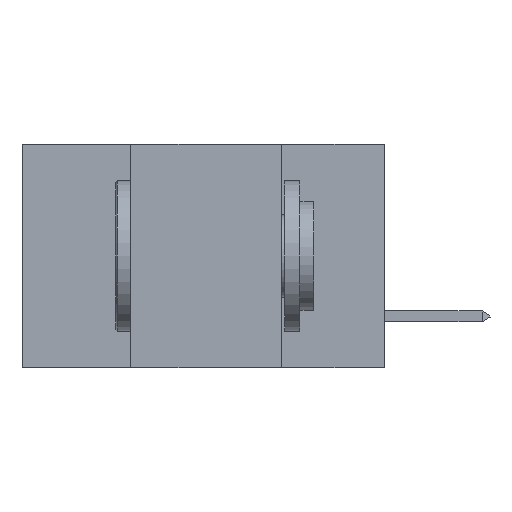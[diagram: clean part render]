
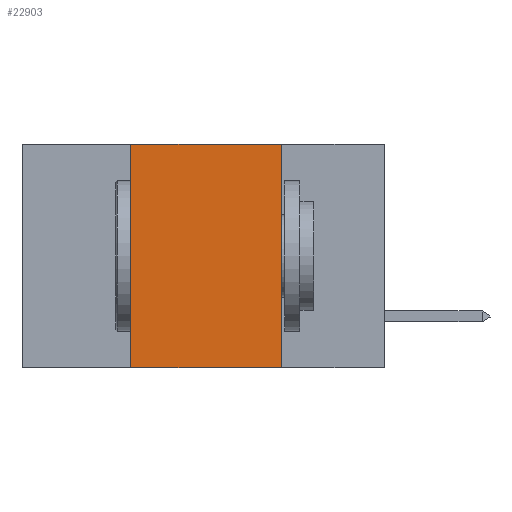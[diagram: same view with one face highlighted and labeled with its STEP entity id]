
A CAD part, left-side view. The second image highlights one B-rep face of the part: STEP entity #22903.
In plain terms, the highlighted planar face has unit normal (-1, 0, 0).
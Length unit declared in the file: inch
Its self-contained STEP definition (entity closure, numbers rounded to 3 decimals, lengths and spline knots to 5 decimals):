
#1036 = DIRECTION ( 'NONE',  ( 0., 0., -1. ) ) ;
#1181 = ORIENTED_EDGE ( 'NONE', *, *, #3146, .T. ) ;
#2586 = CARTESIAN_POINT ( 'NONE',  ( 0., 0.6, 0. ) ) ;
#2651 = CARTESIAN_POINT ( 'NONE',  ( 0., 0.17, -0.37 ) ) ;
#3146 = EDGE_CURVE ( 'NONE', #17203, #20157, #23540, .T. ) ;
#3471 = CARTESIAN_POINT ( 'NONE',  ( 0., 0.42, 0. ) ) ;
#3486 = VERTEX_POINT ( 'NONE', #8596 ) ;
#3766 = ORIENTED_EDGE ( 'NONE', *, *, #17539, .F. ) ;
#3895 = EDGE_LOOP ( 'NONE', ( #9878, #3766, #4233, #1181 ) ) ;
#4100 = CARTESIAN_POINT ( 'NONE',  ( 0., 0.42, -0.37 ) ) ;
#4233 = ORIENTED_EDGE ( 'NONE', *, *, #4370, .F. ) ;
#4370 = EDGE_CURVE ( 'NONE', #17203, #14388, #13505, .T. ) ;
#5021 = DIRECTION ( 'NONE',  ( 0., 0., -1. ) ) ;
#5562 = EDGE_CURVE ( 'NONE', #3486, #20157, #23439, .T. ) ;
#8101 = DIRECTION ( 'NONE',  ( 0., -1., 0. ) ) ;
#8596 = CARTESIAN_POINT ( 'NONE',  ( 0., 0.17, 0. ) ) ;
#8772 = VECTOR ( 'NONE', #1036, 39.37008 ) ;
#8903 = DIRECTION ( 'NONE',  ( 1., 0., 0. ) ) ;
#9878 = ORIENTED_EDGE ( 'NONE', *, *, #5562, .F. ) ;
#10822 = PLANE ( 'NONE',  #22894 ) ;
#12087 = CARTESIAN_POINT ( 'NONE',  ( 0., 0.17, 0. ) ) ;
#12493 = DIRECTION ( 'NONE',  ( 0., 0., 1. ) ) ;
#13505 = LINE ( 'NONE', #3471, #13774 ) ;
#13774 = VECTOR ( 'NONE', #12493, 39.37008 ) ;
#14388 = VERTEX_POINT ( 'NONE', #16921 ) ;
#15476 = CARTESIAN_POINT ( 'NONE',  ( 0., 0.6, -0.37 ) ) ;
#16921 = CARTESIAN_POINT ( 'NONE',  ( 0., 0.42, 0. ) ) ;
#17203 = VERTEX_POINT ( 'NONE', #4100 ) ;
#17539 = EDGE_CURVE ( 'NONE', #14388, #3486, #21039, .T. ) ;
#18882 = FACE_OUTER_BOUND ( 'NONE', #3895, .T. ) ;
#19045 = VECTOR ( 'NONE', #23107, 39.37008 ) ;
#20157 = VERTEX_POINT ( 'NONE', #2651 ) ;
#21039 = LINE ( 'NONE', #2586, #19045 ) ;
#21231 = VECTOR ( 'NONE', #8101, 39.37008 ) ;
#22894 = AXIS2_PLACEMENT_3D ( 'NONE', #23543, #8903, #5021 ) ;
#22903 = ADVANCED_FACE ( 'NONE', ( #18882 ), #10822, .F. ) ;
#23107 = DIRECTION ( 'NONE',  ( 0., -1., 0. ) ) ;
#23439 = LINE ( 'NONE', #12087, #8772 ) ;
#23540 = LINE ( 'NONE', #15476, #21231 ) ;
#23543 = CARTESIAN_POINT ( 'NONE',  ( 0., 0.6, 0. ) ) ;
